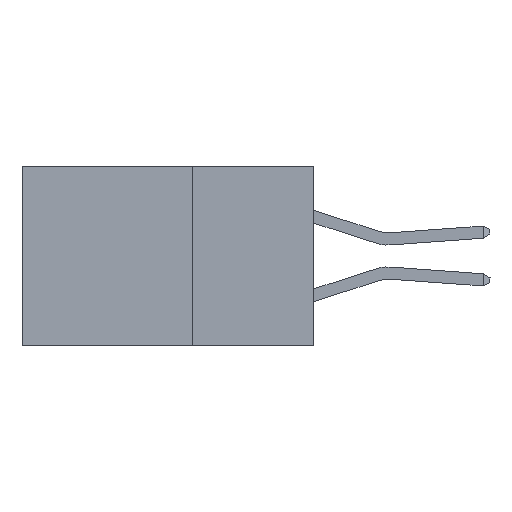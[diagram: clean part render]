
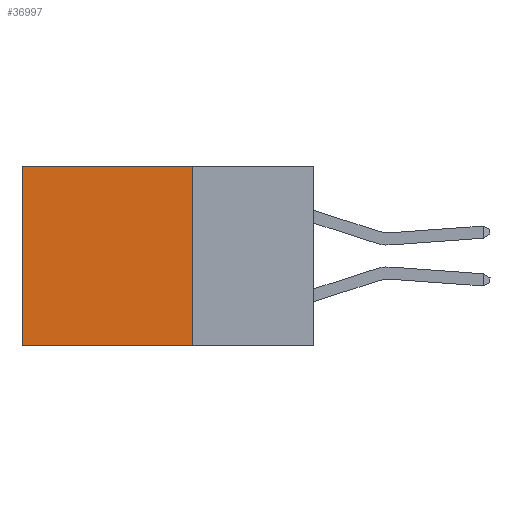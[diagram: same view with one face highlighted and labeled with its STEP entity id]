
A CAD part, left-side view. The second image highlights one B-rep face of the part: STEP entity #36997.
In plain terms, the highlighted planar face has unit normal (-1, 0, 0).
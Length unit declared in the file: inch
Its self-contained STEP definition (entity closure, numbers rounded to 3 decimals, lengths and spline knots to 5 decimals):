
#780 = DIRECTION ( 'NONE',  ( 0., 1., 0. ) ) ;
#2621 = EDGE_CURVE ( 'NONE', #27872, #28215, #26336, .T. ) ;
#3123 = EDGE_CURVE ( 'NONE', #20580, #28215, #23381, .T. ) ;
#3130 = ORIENTED_EDGE ( 'NONE', *, *, #19816, .F. ) ;
#3652 = VECTOR ( 'NONE', #24946, 39.37008 ) ;
#4917 = DIRECTION ( 'NONE',  ( 0., 0., -1. ) ) ;
#5522 = LINE ( 'NONE', #40420, #38558 ) ;
#5899 = CARTESIAN_POINT ( 'NONE',  ( 0.2875, 0.25, -0.37 ) ) ;
#7066 = ORIENTED_EDGE ( 'NONE', *, *, #36202, .T. ) ;
#10273 = DIRECTION ( 'NONE',  ( 0., 0., -1. ) ) ;
#10502 = CARTESIAN_POINT ( 'NONE',  ( 0.2875, 0.6, -0.37 ) ) ;
#11435 = FACE_OUTER_BOUND ( 'NONE', #40317, .T. ) ;
#18926 = ORIENTED_EDGE ( 'NONE', *, *, #2621, .T. ) ;
#19741 = DIRECTION ( 'NONE',  ( 1., 0., 0. ) ) ;
#19816 = EDGE_CURVE ( 'NONE', #36139, #20580, #5522, .T. ) ;
#20580 = VERTEX_POINT ( 'NONE', #5899 ) ;
#21212 = DIRECTION ( 'NONE',  ( 0., 0., -1. ) ) ;
#22811 = LINE ( 'NONE', #35382, #28745 ) ;
#23381 = LINE ( 'NONE', #37619, #3652 ) ;
#24946 = DIRECTION ( 'NONE',  ( 0., 1., 0. ) ) ;
#26336 = LINE ( 'NONE', #33416, #34181 ) ;
#27872 = VERTEX_POINT ( 'NONE', #28260 ) ;
#28215 = VERTEX_POINT ( 'NONE', #10502 ) ;
#28260 = CARTESIAN_POINT ( 'NONE',  ( 0.2875, 0.6, 0. ) ) ;
#28713 = PLANE ( 'NONE',  #29217 ) ;
#28745 = VECTOR ( 'NONE', #780, 39.37008 ) ;
#29217 = AXIS2_PLACEMENT_3D ( 'NONE', #35035, #19741, #10273 ) ;
#33416 = CARTESIAN_POINT ( 'NONE',  ( 0.2875, 0.6, 0. ) ) ;
#34181 = VECTOR ( 'NONE', #4917, 39.37008 ) ;
#35035 = CARTESIAN_POINT ( 'NONE',  ( 0.2875, 0.25, 0. ) ) ;
#35382 = CARTESIAN_POINT ( 'NONE',  ( 0.2875, 0.25, 0. ) ) ;
#36139 = VERTEX_POINT ( 'NONE', #37366 ) ;
#36202 = EDGE_CURVE ( 'NONE', #36139, #27872, #22811, .T. ) ;
#36997 = ADVANCED_FACE ( 'NONE', ( #11435 ), #28713, .F. ) ;
#37366 = CARTESIAN_POINT ( 'NONE',  ( 0.2875, 0.25, 0. ) ) ;
#37619 = CARTESIAN_POINT ( 'NONE',  ( 0.2875, 0.25, -0.37 ) ) ;
#38558 = VECTOR ( 'NONE', #21212, 39.37008 ) ;
#39355 = ORIENTED_EDGE ( 'NONE', *, *, #3123, .F. ) ;
#40317 = EDGE_LOOP ( 'NONE', ( #18926, #39355, #3130, #7066 ) ) ;
#40420 = CARTESIAN_POINT ( 'NONE',  ( 0.2875, 0.25, 0. ) ) ;
